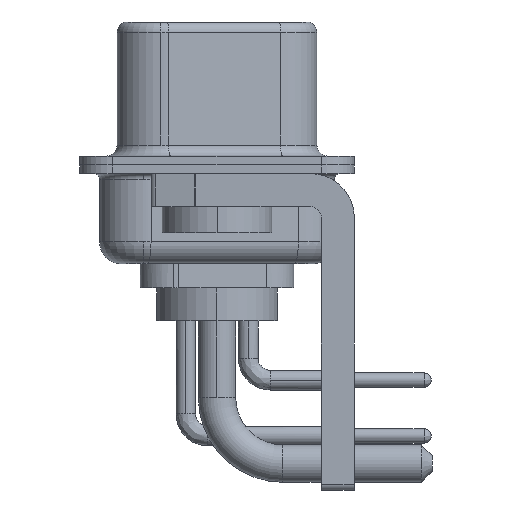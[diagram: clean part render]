
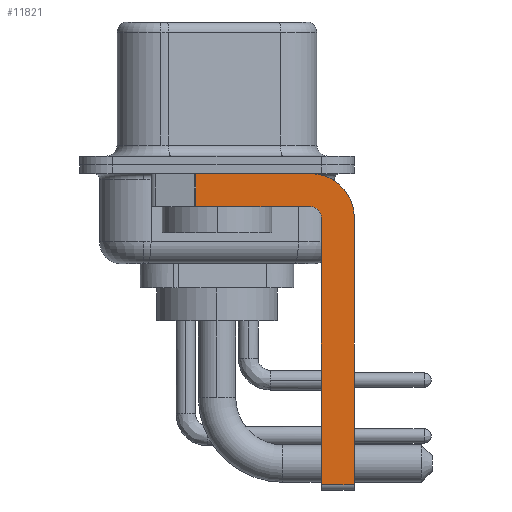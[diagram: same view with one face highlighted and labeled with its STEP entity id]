
A CAD part, left-side view. The second image highlights one B-rep face of the part: STEP entity #11821.
In plain terms, the highlighted planar face has unit normal (-1, 0, 0).
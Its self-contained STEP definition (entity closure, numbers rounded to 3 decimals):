
#1869 = CIRCLE ( 'NONE', #2222, 0.5 ) ;
#2222 = AXIS2_PLACEMENT_3D ( 'NONE', #16037, #19335, #21130 ) ;
#2733 = ORIENTED_EDGE ( 'NONE', *, *, #12004, .F. ) ;
#2928 = CIRCLE ( 'NONE', #20224, 2. ) ;
#3231 = CARTESIAN_POINT ( 'NONE',  ( -2.9, -4.25, -2.4 ) ) ;
#3558 = DIRECTION ( 'NONE',  ( 0., 0., -1. ) ) ;
#3564 = VERTEX_POINT ( 'NONE', #9580 ) ;
#3691 = CARTESIAN_POINT ( 'NONE',  ( -2.9, -4.25, -1.9 ) ) ;
#4329 = CARTESIAN_POINT ( 'NONE',  ( -2.9, -6.25, -2.4 ) ) ;
#4436 = VERTEX_POINT ( 'NONE', #15917 ) ;
#5129 = CARTESIAN_POINT ( 'NONE',  ( -2.9, -4.25, -2.4 ) ) ;
#5645 = ORIENTED_EDGE ( 'NONE', *, *, #21383, .F. ) ;
#6333 = FACE_OUTER_BOUND ( 'NONE', #20668, .T. ) ;
#6592 = EDGE_CURVE ( 'NONE', #4436, #14851, #12167, .T. ) ;
#6621 = VERTEX_POINT ( 'NONE', #15593 ) ;
#6874 = ORIENTED_EDGE ( 'NONE', *, *, #18193, .F. ) ;
#7105 = DIRECTION ( 'NONE',  ( 0., 1., 0. ) ) ;
#7245 = LINE ( 'NONE', #13987, #9074 ) ;
#8702 = LINE ( 'NONE', #17277, #14683 ) ;
#9074 = VECTOR ( 'NONE', #20633, 1000. ) ;
#9209 = ORIENTED_EDGE ( 'NONE', *, *, #15085, .F. ) ;
#9297 = ORIENTED_EDGE ( 'NONE', *, *, #17861, .T. ) ;
#9580 = CARTESIAN_POINT ( 'NONE',  ( -2.9, -4.75, -2.4 ) ) ;
#10234 = CARTESIAN_POINT ( 'NONE',  ( -2.9, -4.75, -14.55 ) ) ;
#11314 = CARTESIAN_POINT ( 'NONE',  ( -2.9, -4.25, -14.55 ) ) ;
#11531 = LINE ( 'NONE', #11314, #16900 ) ;
#11650 = DIRECTION ( 'NONE',  ( 0., 0., -1. ) ) ;
#11747 = DIRECTION ( 'NONE',  ( 0., -1., 0. ) ) ;
#11821 = ADVANCED_FACE ( 'NONE', ( #6333 ), #16837, .F. ) ;
#12004 = EDGE_CURVE ( 'NONE', #3564, #13846, #1869, .T. ) ;
#12104 = DIRECTION ( 'NONE',  ( 0., -1., 0. ) ) ;
#12114 = ORIENTED_EDGE ( 'NONE', *, *, #15846, .F. ) ;
#12167 = LINE ( 'NONE', #17232, #15835 ) ;
#12579 = CARTESIAN_POINT ( 'NONE',  ( -2.9, -4.25, -1.9 ) ) ;
#13523 = DIRECTION ( 'NONE',  ( 1., 0., 0. ) ) ;
#13711 = DIRECTION ( 'NONE',  ( 1., 0., 0. ) ) ;
#13846 = VERTEX_POINT ( 'NONE', #12579 ) ;
#13987 = CARTESIAN_POINT ( 'NONE',  ( -2.9, -4.75, -14.8 ) ) ;
#14648 = EDGE_CURVE ( 'NONE', #4436, #20033, #8702, .T. ) ;
#14683 = VECTOR ( 'NONE', #12104, 1000. ) ;
#14851 = VERTEX_POINT ( 'NONE', #16610 ) ;
#15085 = EDGE_CURVE ( 'NONE', #13846, #14851, #19019, .T. ) ;
#15282 = DIRECTION ( 'NONE',  ( 0., 0., -1. ) ) ;
#15593 = CARTESIAN_POINT ( 'NONE',  ( -2.9, -6.25, -14.55 ) ) ;
#15835 = VECTOR ( 'NONE', #15282, 1000. ) ;
#15846 = EDGE_CURVE ( 'NONE', #16212, #3564, #7245, .T. ) ;
#15917 = CARTESIAN_POINT ( 'NONE',  ( -2.9, 0.978, -0.4 ) ) ;
#16037 = CARTESIAN_POINT ( 'NONE',  ( -2.9, -4.25, -2.4 ) ) ;
#16212 = VERTEX_POINT ( 'NONE', #10234 ) ;
#16381 = CARTESIAN_POINT ( 'NONE',  ( -2.9, -6.25, -2.4 ) ) ;
#16448 = VERTEX_POINT ( 'NONE', #16381 ) ;
#16610 = CARTESIAN_POINT ( 'NONE',  ( -2.9, 0.978, -1.9 ) ) ;
#16837 = PLANE ( 'NONE',  #20628 ) ;
#16900 = VECTOR ( 'NONE', #11747, 1000. ) ;
#17232 = CARTESIAN_POINT ( 'NONE',  ( -2.9, 0.978, -1.9 ) ) ;
#17277 = CARTESIAN_POINT ( 'NONE',  ( -2.9, 3., -0.4 ) ) ;
#17861 = EDGE_CURVE ( 'NONE', #16212, #6621, #11531, .T. ) ;
#18193 = EDGE_CURVE ( 'NONE', #16448, #6621, #19572, .T. ) ;
#19019 = LINE ( 'NONE', #3691, #19254 ) ;
#19233 = DIRECTION ( 'NONE',  ( 0., 0., -1. ) ) ;
#19254 = VECTOR ( 'NONE', #7105, 1000. ) ;
#19335 = DIRECTION ( 'NONE',  ( -1., 0., 0. ) ) ;
#19465 = CARTESIAN_POINT ( 'NONE',  ( -2.9, -4.25, -0.4 ) ) ;
#19510 = ORIENTED_EDGE ( 'NONE', *, *, #14648, .F. ) ;
#19572 = LINE ( 'NONE', #4329, #21527 ) ;
#20033 = VERTEX_POINT ( 'NONE', #19465 ) ;
#20224 = AXIS2_PLACEMENT_3D ( 'NONE', #3231, #13711, #3558 ) ;
#20628 = AXIS2_PLACEMENT_3D ( 'NONE', #5129, #13523, #11650 ) ;
#20633 = DIRECTION ( 'NONE',  ( 0., 0., 1. ) ) ;
#20668 = EDGE_LOOP ( 'NONE', ( #19510, #21814, #9209, #2733, #12114, #9297, #6874, #5645 ) ) ;
#21130 = DIRECTION ( 'NONE',  ( 0., 0., 1. ) ) ;
#21383 = EDGE_CURVE ( 'NONE', #20033, #16448, #2928, .T. ) ;
#21527 = VECTOR ( 'NONE', #19233, 1000. ) ;
#21814 = ORIENTED_EDGE ( 'NONE', *, *, #6592, .T. ) ;
